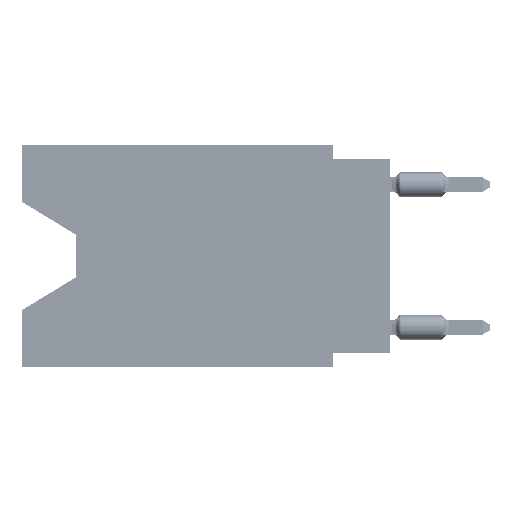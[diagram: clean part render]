
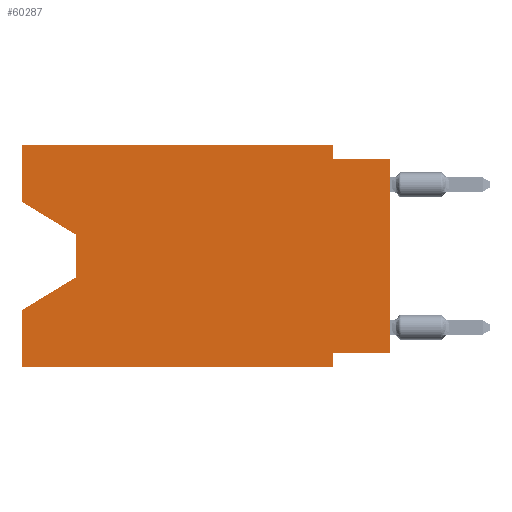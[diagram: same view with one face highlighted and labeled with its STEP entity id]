
A CAD part, left-side view. The second image highlights one B-rep face of the part: STEP entity #60287.
In plain terms, the highlighted planar face has unit normal (-1, 0, 0).
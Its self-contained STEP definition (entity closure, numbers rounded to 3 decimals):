
#172 = EDGE_CURVE ( 'NONE', #21646, #27518, #22687, .T. ) ;
#460 = EDGE_CURVE ( 'NONE', #538, #15277, #4405, .T. ) ;
#538 = VERTEX_POINT ( 'NONE', #34643 ) ;
#649 = CARTESIAN_POINT ( 'NONE',  ( 0., 0., -0.635 ) ) ;
#1433 = VECTOR ( 'NONE', #57769, 1000. ) ;
#1741 = ORIENTED_EDGE ( 'NONE', *, *, #57577, .T. ) ;
#2703 = CARTESIAN_POINT ( 'NONE',  ( 0., 16.383, 0. ) ) ;
#2771 = LINE ( 'NONE', #24990, #68156 ) ;
#3723 = VECTOR ( 'NONE', #69765, 1000. ) ;
#4405 = LINE ( 'NONE', #71449, #44195 ) ;
#5164 = EDGE_CURVE ( 'NONE', #538, #25376, #64162, .T. ) ;
#5201 = VERTEX_POINT ( 'NONE', #47032 ) ;
#7225 = ORIENTED_EDGE ( 'NONE', *, *, #17304, .T. ) ;
#7318 = EDGE_CURVE ( 'NONE', #48793, #41175, #2771, .T. ) ;
#7865 = LINE ( 'NONE', #35230, #28132 ) ;
#8392 = CARTESIAN_POINT ( 'NONE',  ( 0., 2.54, -9.906 ) ) ;
#8788 = EDGE_LOOP ( 'NONE', ( #56219, #1741, #7225, #12260, #62939, #36286, #20432, #28676, #20300, #59982, #68863, #28748 ) ) ;
#12260 = ORIENTED_EDGE ( 'NONE', *, *, #172, .F. ) ;
#13483 = CARTESIAN_POINT ( 'NONE',  ( 0., 16.383, -2.546 ) ) ;
#15277 = VERTEX_POINT ( 'NONE', #23163 ) ;
#15818 = LINE ( 'NONE', #71972, #49179 ) ;
#16329 = CARTESIAN_POINT ( 'NONE',  ( 0., 2.54, -9.271 ) ) ;
#17003 = EDGE_CURVE ( 'NONE', #35667, #35591, #46267, .T. ) ;
#17304 = EDGE_CURVE ( 'NONE', #5201, #27518, #63575, .T. ) ;
#18317 = CARTESIAN_POINT ( 'NONE',  ( 0., 2.54, 0. ) ) ;
#18727 = EDGE_CURVE ( 'NONE', #19649, #35667, #15818, .T. ) ;
#18762 = LINE ( 'NONE', #67998, #1433 ) ;
#19222 = VECTOR ( 'NONE', #30622, 1000. ) ;
#19649 = VERTEX_POINT ( 'NONE', #52125 ) ;
#20097 = DIRECTION ( 'NONE',  ( 0., 0., 1. ) ) ;
#20300 = ORIENTED_EDGE ( 'NONE', *, *, #64575, .F. ) ;
#20432 = ORIENTED_EDGE ( 'NONE', *, *, #18727, .F. ) ;
#21646 = VERTEX_POINT ( 'NONE', #68020 ) ;
#22687 = LINE ( 'NONE', #56597, #39527 ) ;
#22749 = FACE_OUTER_BOUND ( 'NONE', #8788, .T. ) ;
#23163 = CARTESIAN_POINT ( 'NONE',  ( 0., 16.383, 0. ) ) ;
#23685 = CARTESIAN_POINT ( 'NONE',  ( 0., 13.97, -4.013 ) ) ;
#24211 = CARTESIAN_POINT ( 'NONE',  ( 0., 13.97, -5.893 ) ) ;
#24917 = DIRECTION ( 'NONE',  ( 0., 0., -1. ) ) ;
#24990 = CARTESIAN_POINT ( 'NONE',  ( 0., 2.54, 0. ) ) ;
#25376 = VERTEX_POINT ( 'NONE', #23685 ) ;
#27496 = CARTESIAN_POINT ( 'NONE',  ( 0., 16.383, -9.906 ) ) ;
#27518 = VERTEX_POINT ( 'NONE', #49109 ) ;
#28132 = VECTOR ( 'NONE', #51264, 1000. ) ;
#28342 = LINE ( 'NONE', #649, #62615 ) ;
#28676 = ORIENTED_EDGE ( 'NONE', *, *, #47197, .T. ) ;
#28748 = ORIENTED_EDGE ( 'NONE', *, *, #460, .F. ) ;
#28871 = VERTEX_POINT ( 'NONE', #71428 ) ;
#29844 = CARTESIAN_POINT ( 'NONE',  ( 0., 2.54, -9.906 ) ) ;
#30622 = DIRECTION ( 'NONE',  ( 0., -0.855, -0.519 ) ) ;
#31340 = LINE ( 'NONE', #64505, #70216 ) ;
#34643 = CARTESIAN_POINT ( 'NONE',  ( 0., 16.383, -2.546 ) ) ;
#35230 = CARTESIAN_POINT ( 'NONE',  ( 0., 13.97, -4.013 ) ) ;
#35519 = DIRECTION ( 'NONE',  ( 1., 0., 0. ) ) ;
#35591 = VERTEX_POINT ( 'NONE', #8392 ) ;
#35667 = VERTEX_POINT ( 'NONE', #16329 ) ;
#36286 = ORIENTED_EDGE ( 'NONE', *, *, #17003, .F. ) ;
#37167 = DIRECTION ( 'NONE',  ( 0., -1., 0. ) ) ;
#38462 = DIRECTION ( 'NONE',  ( 0., -1., 0. ) ) ;
#39527 = VECTOR ( 'NONE', #20097, 1000. ) ;
#41175 = VERTEX_POINT ( 'NONE', #59144 ) ;
#44195 = VECTOR ( 'NONE', #70400, 1000. ) ;
#46267 = LINE ( 'NONE', #29844, #63054 ) ;
#47032 = CARTESIAN_POINT ( 'NONE',  ( 0., 13.97, -5.893 ) ) ;
#47197 = EDGE_CURVE ( 'NONE', #19649, #28871, #18762, .T. ) ;
#48156 = EDGE_CURVE ( 'NONE', #15277, #48793, #31340, .T. ) ;
#48676 = LINE ( 'NONE', #27496, #64590 ) ;
#48793 = VERTEX_POINT ( 'NONE', #18317 ) ;
#49109 = CARTESIAN_POINT ( 'NONE',  ( 0., 16.383, -7.36 ) ) ;
#49179 = VECTOR ( 'NONE', #66170, 1000. ) ;
#51264 = DIRECTION ( 'NONE',  ( 0., 0., -1. ) ) ;
#51671 = DIRECTION ( 'NONE',  ( 0., -1., 0. ) ) ;
#52125 = CARTESIAN_POINT ( 'NONE',  ( 0., 0., -9.271 ) ) ;
#56219 = ORIENTED_EDGE ( 'NONE', *, *, #5164, .T. ) ;
#56597 = CARTESIAN_POINT ( 'NONE',  ( 0., 16.383, 0. ) ) ;
#57454 = DIRECTION ( 'NONE',  ( 0., 0., -1. ) ) ;
#57577 = EDGE_CURVE ( 'NONE', #25376, #5201, #7865, .T. ) ;
#57769 = DIRECTION ( 'NONE',  ( 0., 0., 1. ) ) ;
#59144 = CARTESIAN_POINT ( 'NONE',  ( 0., 2.54, -0.635 ) ) ;
#59982 = ORIENTED_EDGE ( 'NONE', *, *, #7318, .F. ) ;
#60287 = ADVANCED_FACE ( 'NONE', ( #22749 ), #61768, .F. ) ;
#61308 = EDGE_CURVE ( 'NONE', #21646, #35591, #48676, .T. ) ;
#61768 = PLANE ( 'NONE',  #71431 ) ;
#62615 = VECTOR ( 'NONE', #51671, 1000. ) ;
#62939 = ORIENTED_EDGE ( 'NONE', *, *, #61308, .T. ) ;
#63054 = VECTOR ( 'NONE', #65178, 1000. ) ;
#63575 = LINE ( 'NONE', #24211, #3723 ) ;
#64162 = LINE ( 'NONE', #13483, #19222 ) ;
#64505 = CARTESIAN_POINT ( 'NONE',  ( 0., 16.383, 0. ) ) ;
#64575 = EDGE_CURVE ( 'NONE', #41175, #28871, #28342, .T. ) ;
#64590 = VECTOR ( 'NONE', #38462, 1000. ) ;
#65178 = DIRECTION ( 'NONE',  ( 0., 0., -1. ) ) ;
#66170 = DIRECTION ( 'NONE',  ( 0., 1., 0. ) ) ;
#67998 = CARTESIAN_POINT ( 'NONE',  ( 0., 0., 0. ) ) ;
#68020 = CARTESIAN_POINT ( 'NONE',  ( 0., 16.383, -9.906 ) ) ;
#68156 = VECTOR ( 'NONE', #57454, 1000. ) ;
#68863 = ORIENTED_EDGE ( 'NONE', *, *, #48156, .F. ) ;
#69765 = DIRECTION ( 'NONE',  ( 0., 0.855, -0.519 ) ) ;
#70216 = VECTOR ( 'NONE', #37167, 1000. ) ;
#70400 = DIRECTION ( 'NONE',  ( 0., 0., 1. ) ) ;
#71428 = CARTESIAN_POINT ( 'NONE',  ( 0., 0., -0.635 ) ) ;
#71431 = AXIS2_PLACEMENT_3D ( 'NONE', #2703, #35519, #24917 ) ;
#71449 = CARTESIAN_POINT ( 'NONE',  ( 0., 16.383, 0. ) ) ;
#71972 = CARTESIAN_POINT ( 'NONE',  ( 0., 0., -9.271 ) ) ;
